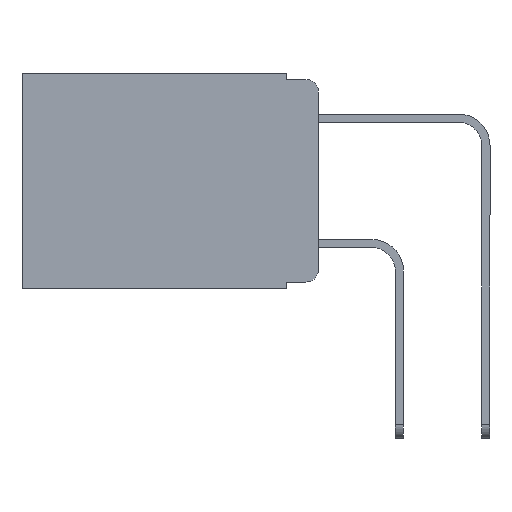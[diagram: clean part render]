
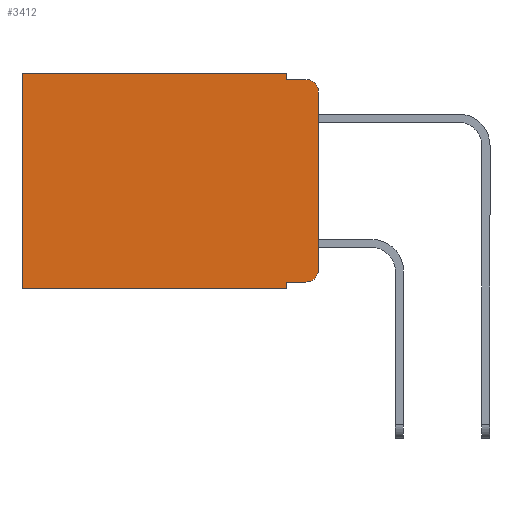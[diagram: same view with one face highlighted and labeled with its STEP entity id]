
A CAD part, left-side view. The second image highlights one B-rep face of the part: STEP entity #3412.
In plain terms, the highlighted planar face has unit normal (-1, 0, 0).
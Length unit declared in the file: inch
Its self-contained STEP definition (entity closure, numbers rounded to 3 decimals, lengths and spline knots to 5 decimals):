
#101 = LINE ( 'NONE', #9946, #6817 ) ;
#113 = CARTESIAN_POINT ( 'NONE',  ( 0.298, 0.051, 0. ) ) ;
#114 = FACE_OUTER_BOUND ( 'NONE', #9036, .T. ) ;
#150 = DIRECTION ( 'NONE',  ( 0., 0., -1. ) ) ;
#223 = EDGE_CURVE ( 'NONE', #10470, #2496, #9105, .T. ) ;
#464 = VECTOR ( 'NONE', #2321, 39.37008 ) ;
#518 = VERTEX_POINT ( 'NONE', #1749 ) ;
#620 = VECTOR ( 'NONE', #150, 39.37008 ) ;
#745 = VERTEX_POINT ( 'NONE', #3173 ) ;
#767 = LINE ( 'NONE', #1406, #464 ) ;
#871 = ORIENTED_EDGE ( 'NONE', *, *, #7125, .F. ) ;
#1081 = CARTESIAN_POINT ( 'NONE',  ( 0.298, 0., -0.343 ) ) ;
#1145 = ORIENTED_EDGE ( 'NONE', *, *, #3993, .F. ) ;
#1406 = CARTESIAN_POINT ( 'NONE',  ( 0.298, 0., 0. ) ) ;
#1483 = LINE ( 'NONE', #8407, #8128 ) ;
#1569 = DIRECTION ( 'NONE',  ( 0., 0., -1. ) ) ;
#1749 = CARTESIAN_POINT ( 'NONE',  ( 0.298, 0.051, -0.343 ) ) ;
#1908 = CARTESIAN_POINT ( 'NONE',  ( 0.298, 0.051, 0. ) ) ;
#2321 = DIRECTION ( 'NONE',  ( 0., 1., 0. ) ) ;
#2496 = VERTEX_POINT ( 'NONE', #2884 ) ;
#2529 = VERTEX_POINT ( 'NONE', #2671 ) ;
#2642 = LINE ( 'NONE', #6328, #7212 ) ;
#2671 = CARTESIAN_POINT ( 'NONE',  ( 0.298, 0.051, -0.01 ) ) ;
#2884 = CARTESIAN_POINT ( 'NONE',  ( 0.298, 0.02, -0.01 ) ) ;
#3173 = CARTESIAN_POINT ( 'NONE',  ( 0.298, 0., -0.313 ) ) ;
#3364 = LINE ( 'NONE', #10179, #8092 ) ;
#3412 = ADVANCED_FACE ( 'NONE', ( #114 ), #9604, .F. ) ;
#3833 = EDGE_CURVE ( 'NONE', #9009, #745, #5976, .T. ) ;
#3993 = EDGE_CURVE ( 'NONE', #10470, #745, #4339, .T. ) ;
#4049 = VECTOR ( 'NONE', #5910, 39.37008 ) ;
#4065 = CARTESIAN_POINT ( 'NONE',  ( 0.298, 0.02, -0.03 ) ) ;
#4339 = LINE ( 'NONE', #10123, #4049 ) ;
#4364 = AXIS2_PLACEMENT_3D ( 'NONE', #5497, #11387, #6381 ) ;
#5097 = DIRECTION ( 'NONE',  ( 0., -1., 0. ) ) ;
#5156 = CARTESIAN_POINT ( 'NONE',  ( 0.298, 0.473, -0.343 ) ) ;
#5218 = AXIS2_PLACEMENT_3D ( 'NONE', #4065, #6774, #8774 ) ;
#5228 = CARTESIAN_POINT ( 'NONE',  ( 0.298, 0.02, -0.333 ) ) ;
#5497 = CARTESIAN_POINT ( 'NONE',  ( 0.298, 0.02, -0.313 ) ) ;
#5910 = DIRECTION ( 'NONE',  ( 0., 0., -1. ) ) ;
#5976 = CIRCLE ( 'NONE', #4364, 0.02 ) ;
#6007 = LINE ( 'NONE', #1081, #10503 ) ;
#6328 = CARTESIAN_POINT ( 'NONE',  ( 0.298, 0.051, 0. ) ) ;
#6381 = DIRECTION ( 'NONE',  ( 0., 0., -1. ) ) ;
#6604 = DIRECTION ( 'NONE',  ( 0., 0., -1. ) ) ;
#6607 = ORIENTED_EDGE ( 'NONE', *, *, #11065, .F. ) ;
#6774 = DIRECTION ( 'NONE',  ( -1., 0., 0. ) ) ;
#6811 = EDGE_CURVE ( 'NONE', #10147, #9009, #3364, .T. ) ;
#6817 = VECTOR ( 'NONE', #6604, 39.37008 ) ;
#7125 = EDGE_CURVE ( 'NONE', #518, #8942, #6007, .T. ) ;
#7212 = VECTOR ( 'NONE', #9689, 39.37008 ) ;
#7416 = CARTESIAN_POINT ( 'NONE',  ( 0.298, 0.051, -0.333 ) ) ;
#7450 = DIRECTION ( 'NONE',  ( 0., 1., 0. ) ) ;
#7628 = ORIENTED_EDGE ( 'NONE', *, *, #3833, .T. ) ;
#7737 = CARTESIAN_POINT ( 'NONE',  ( 0.298, 0., 0. ) ) ;
#8092 = VECTOR ( 'NONE', #5097, 39.37008 ) ;
#8128 = VECTOR ( 'NONE', #10822, 39.37008 ) ;
#8182 = AXIS2_PLACEMENT_3D ( 'NONE', #7737, #9652, #1569 ) ;
#8343 = EDGE_CURVE ( 'NONE', #8566, #8942, #101, .T. ) ;
#8407 = CARTESIAN_POINT ( 'NONE',  ( 0.298, 0.051, -0.01 ) ) ;
#8566 = VERTEX_POINT ( 'NONE', #8581 ) ;
#8581 = CARTESIAN_POINT ( 'NONE',  ( 0.298, 0.473, 0. ) ) ;
#8712 = VERTEX_POINT ( 'NONE', #1908 ) ;
#8774 = DIRECTION ( 'NONE',  ( 0., 0., -1. ) ) ;
#8942 = VERTEX_POINT ( 'NONE', #5156 ) ;
#9009 = VERTEX_POINT ( 'NONE', #5228 ) ;
#9036 = EDGE_LOOP ( 'NONE', ( #1145, #9370, #6607, #10523, #9620, #11031, #871, #10910, #10164, #7628 ) ) ;
#9105 = CIRCLE ( 'NONE', #5218, 0.02 ) ;
#9370 = ORIENTED_EDGE ( 'NONE', *, *, #223, .T. ) ;
#9604 = PLANE ( 'NONE',  #8182 ) ;
#9620 = ORIENTED_EDGE ( 'NONE', *, *, #10388, .T. ) ;
#9652 = DIRECTION ( 'NONE',  ( 1., 0., 0. ) ) ;
#9689 = DIRECTION ( 'NONE',  ( 0., 0., -1. ) ) ;
#9946 = CARTESIAN_POINT ( 'NONE',  ( 0.298, 0.473, 0. ) ) ;
#9976 = EDGE_CURVE ( 'NONE', #8712, #2529, #2642, .T. ) ;
#10054 = LINE ( 'NONE', #113, #620 ) ;
#10123 = CARTESIAN_POINT ( 'NONE',  ( 0.298, 0., 0. ) ) ;
#10147 = VERTEX_POINT ( 'NONE', #7416 ) ;
#10161 = EDGE_CURVE ( 'NONE', #10147, #518, #10054, .T. ) ;
#10164 = ORIENTED_EDGE ( 'NONE', *, *, #6811, .T. ) ;
#10179 = CARTESIAN_POINT ( 'NONE',  ( 0.298, 0.051, -0.333 ) ) ;
#10388 = EDGE_CURVE ( 'NONE', #8712, #8566, #767, .T. ) ;
#10470 = VERTEX_POINT ( 'NONE', #11077 ) ;
#10503 = VECTOR ( 'NONE', #7450, 39.37008 ) ;
#10523 = ORIENTED_EDGE ( 'NONE', *, *, #9976, .F. ) ;
#10822 = DIRECTION ( 'NONE',  ( 0., -1., 0. ) ) ;
#10910 = ORIENTED_EDGE ( 'NONE', *, *, #10161, .F. ) ;
#11031 = ORIENTED_EDGE ( 'NONE', *, *, #8343, .T. ) ;
#11065 = EDGE_CURVE ( 'NONE', #2529, #2496, #1483, .T. ) ;
#11077 = CARTESIAN_POINT ( 'NONE',  ( 0.298, 0., -0.03 ) ) ;
#11387 = DIRECTION ( 'NONE',  ( -1., 0., 0. ) ) ;
